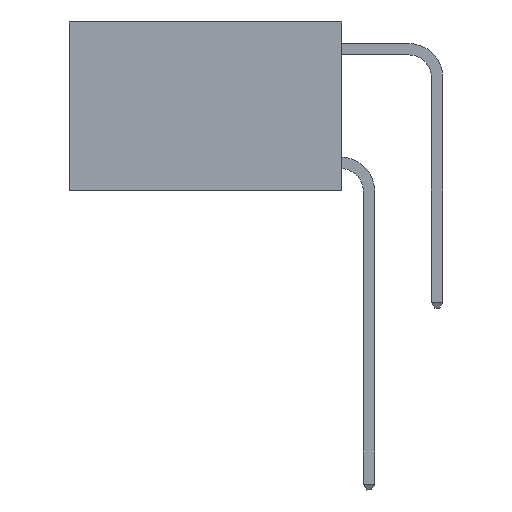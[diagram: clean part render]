
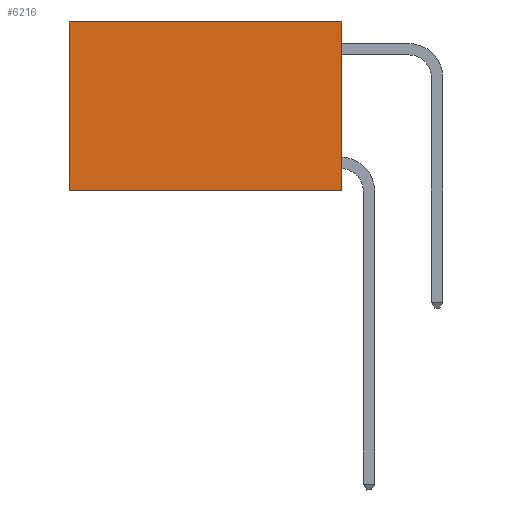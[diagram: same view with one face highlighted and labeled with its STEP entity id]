
A CAD part, left-side view. The second image highlights one B-rep face of the part: STEP entity #6216.
In plain terms, the highlighted planar face has unit normal (-1, 0, 0).
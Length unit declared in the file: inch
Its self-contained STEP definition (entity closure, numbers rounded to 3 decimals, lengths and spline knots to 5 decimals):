
#232 = CARTESIAN_POINT ( 'NONE',  ( 0.2625, 0., 0. ) ) ;
#664 = EDGE_CURVE ( 'NONE', #9541, #2938, #4335, .T. ) ;
#1153 = DIRECTION ( 'NONE',  ( 0., 1., 0. ) ) ;
#1499 = LINE ( 'NONE', #4590, #10387 ) ;
#1551 = LINE ( 'NONE', #232, #10426 ) ;
#1731 = FACE_OUTER_BOUND ( 'NONE', #4713, .T. ) ;
#2843 = VERTEX_POINT ( 'NONE', #7739 ) ;
#2938 = VERTEX_POINT ( 'NONE', #6977 ) ;
#3145 = EDGE_CURVE ( 'NONE', #2843, #9541, #1499, .T. ) ;
#3859 = DIRECTION ( 'NONE',  ( 0., 1., 0. ) ) ;
#4184 = CARTESIAN_POINT ( 'NONE',  ( 0.2625, 0., -0.37 ) ) ;
#4335 = LINE ( 'NONE', #4184, #10819 ) ;
#4357 = VECTOR ( 'NONE', #9364, 39.37008 ) ;
#4377 = DIRECTION ( 'NONE',  ( 0., 0., -1. ) ) ;
#4492 = ORIENTED_EDGE ( 'NONE', *, *, #7620, .T. ) ;
#4547 = ORIENTED_EDGE ( 'NONE', *, *, #3145, .F. ) ;
#4590 = CARTESIAN_POINT ( 'NONE',  ( 0.2625, 0., 0. ) ) ;
#4613 = CARTESIAN_POINT ( 'NONE',  ( 0.2625, 0., 0. ) ) ;
#4713 = EDGE_LOOP ( 'NONE', ( #5110, #7094, #4547, #4492 ) ) ;
#5110 = ORIENTED_EDGE ( 'NONE', *, *, #5334, .T. ) ;
#5334 = EDGE_CURVE ( 'NONE', #7070, #2938, #8705, .T. ) ;
#5546 = DIRECTION ( 'NONE',  ( 0., 0., -1. ) ) ;
#6040 = AXIS2_PLACEMENT_3D ( 'NONE', #4613, #10558, #5546 ) ;
#6216 = ADVANCED_FACE ( 'NONE', ( #1731 ), #9749, .F. ) ;
#6735 = CARTESIAN_POINT ( 'NONE',  ( 0.2625, 0.6, 0. ) ) ;
#6855 = CARTESIAN_POINT ( 'NONE',  ( 0.2625, 0.6, 0. ) ) ;
#6977 = CARTESIAN_POINT ( 'NONE',  ( 0.2625, 0.6, -0.37 ) ) ;
#7070 = VERTEX_POINT ( 'NONE', #6735 ) ;
#7094 = ORIENTED_EDGE ( 'NONE', *, *, #664, .F. ) ;
#7620 = EDGE_CURVE ( 'NONE', #2843, #7070, #1551, .T. ) ;
#7739 = CARTESIAN_POINT ( 'NONE',  ( 0.2625, 0., 0. ) ) ;
#8705 = LINE ( 'NONE', #6855, #4357 ) ;
#9364 = DIRECTION ( 'NONE',  ( 0., 0., -1. ) ) ;
#9541 = VERTEX_POINT ( 'NONE', #9992 ) ;
#9749 = PLANE ( 'NONE',  #6040 ) ;
#9992 = CARTESIAN_POINT ( 'NONE',  ( 0.2625, 0., -0.37 ) ) ;
#10387 = VECTOR ( 'NONE', #4377, 39.37008 ) ;
#10426 = VECTOR ( 'NONE', #1153, 39.37008 ) ;
#10558 = DIRECTION ( 'NONE',  ( 1., 0., 0. ) ) ;
#10819 = VECTOR ( 'NONE', #3859, 39.37008 ) ;
